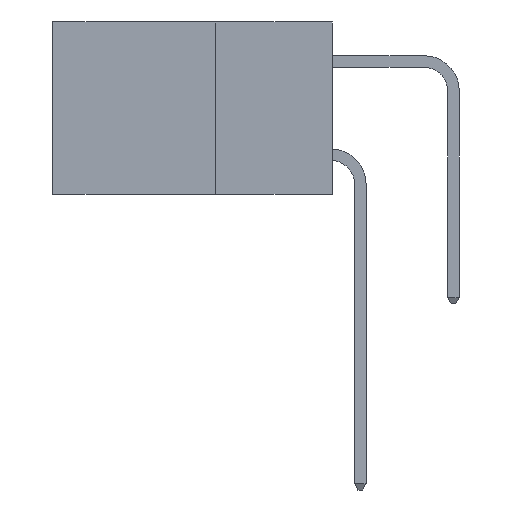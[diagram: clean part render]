
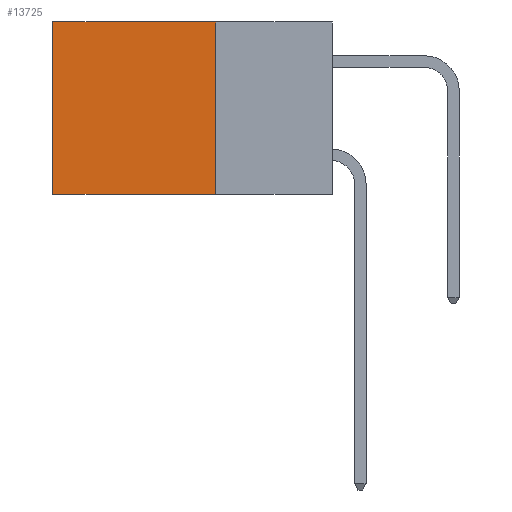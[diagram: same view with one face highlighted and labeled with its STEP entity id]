
A CAD part, left-side view. The second image highlights one B-rep face of the part: STEP entity #13725.
In plain terms, the highlighted planar face has unit normal (-1, 0, 0).
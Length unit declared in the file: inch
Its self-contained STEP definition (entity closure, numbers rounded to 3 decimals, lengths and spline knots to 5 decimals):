
#525 = VERTEX_POINT ( 'NONE', #10009 ) ;
#1497 = LINE ( 'NONE', #4889, #10330 ) ;
#1987 = VERTEX_POINT ( 'NONE', #11273 ) ;
#2141 = VERTEX_POINT ( 'NONE', #6260 ) ;
#2838 = PLANE ( 'NONE',  #4003 ) ;
#3153 = EDGE_CURVE ( 'NONE', #1987, #14085, #1497, .T. ) ;
#3991 = DIRECTION ( 'NONE',  ( 0., 0., -1. ) ) ;
#4003 = AXIS2_PLACEMENT_3D ( 'NONE', #6204, #10512, #3991 ) ;
#4523 = ORIENTED_EDGE ( 'NONE', *, *, #8566, .T. ) ;
#4625 = ORIENTED_EDGE ( 'NONE', *, *, #3153, .F. ) ;
#4765 = VECTOR ( 'NONE', #7606, 39.37008 ) ;
#4887 = DIRECTION ( 'NONE',  ( 0., 1., 0. ) ) ;
#4889 = CARTESIAN_POINT ( 'NONE',  ( 0.2615, 0.25, -0.37 ) ) ;
#5092 = ORIENTED_EDGE ( 'NONE', *, *, #7138, .F. ) ;
#5149 = ORIENTED_EDGE ( 'NONE', *, *, #11271, .T. ) ;
#5781 = LINE ( 'NONE', #12374, #13554 ) ;
#6204 = CARTESIAN_POINT ( 'NONE',  ( 0.2615, 0.25, -0.37 ) ) ;
#6260 = CARTESIAN_POINT ( 'NONE',  ( 0.2615, 0.6, -0.37 ) ) ;
#6717 = CARTESIAN_POINT ( 'NONE',  ( 0.2615, 0.25, -0.37 ) ) ;
#7138 = EDGE_CURVE ( 'NONE', #14085, #2141, #9914, .T. ) ;
#7606 = DIRECTION ( 'NONE',  ( 0., 1., 0. ) ) ;
#8566 = EDGE_CURVE ( 'NONE', #1987, #525, #5781, .T. ) ;
#9277 = DIRECTION ( 'NONE',  ( 0., 0., -1. ) ) ;
#9914 = LINE ( 'NONE', #13849, #4765 ) ;
#10009 = CARTESIAN_POINT ( 'NONE',  ( 0.2615, 0.6, 0. ) ) ;
#10330 = VECTOR ( 'NONE', #9277, 39.37008 ) ;
#10512 = DIRECTION ( 'NONE',  ( 1., 0., 0. ) ) ;
#11014 = FACE_OUTER_BOUND ( 'NONE', #12183, .T. ) ;
#11270 = VECTOR ( 'NONE', #13703, 39.37008 ) ;
#11271 = EDGE_CURVE ( 'NONE', #525, #2141, #13986, .T. ) ;
#11273 = CARTESIAN_POINT ( 'NONE',  ( 0.2615, 0.25, 0. ) ) ;
#12183 = EDGE_LOOP ( 'NONE', ( #5149, #5092, #4625, #4523 ) ) ;
#12374 = CARTESIAN_POINT ( 'NONE',  ( 0.2615, 0.25, 0. ) ) ;
#12667 = CARTESIAN_POINT ( 'NONE',  ( 0.2615, 0.6, -0.37 ) ) ;
#13554 = VECTOR ( 'NONE', #4887, 39.37008 ) ;
#13703 = DIRECTION ( 'NONE',  ( 0., 0., -1. ) ) ;
#13725 = ADVANCED_FACE ( 'NONE', ( #11014 ), #2838, .F. ) ;
#13849 = CARTESIAN_POINT ( 'NONE',  ( 0.2615, 0.25, -0.37 ) ) ;
#13986 = LINE ( 'NONE', #12667, #11270 ) ;
#14085 = VERTEX_POINT ( 'NONE', #6717 ) ;
